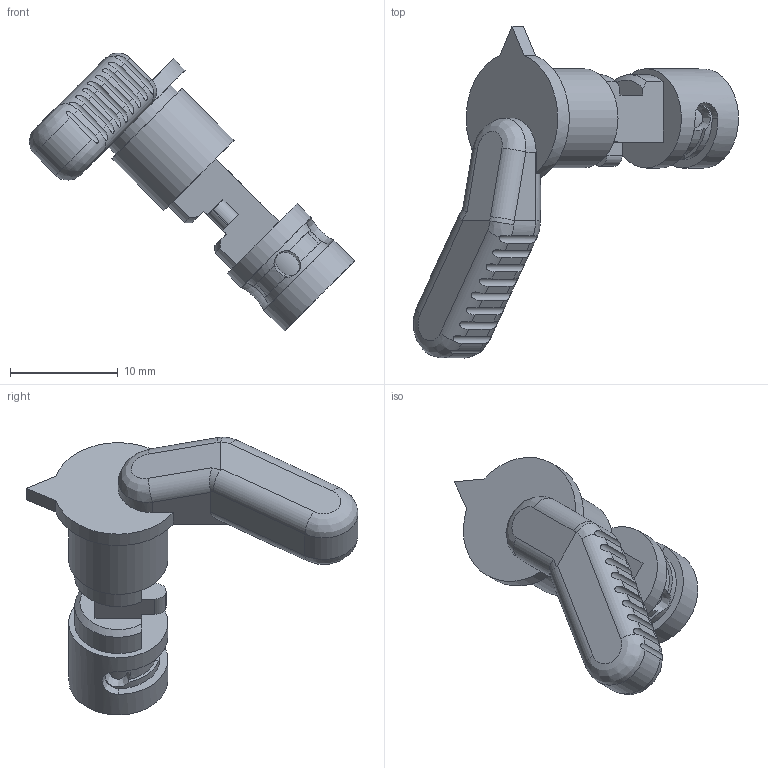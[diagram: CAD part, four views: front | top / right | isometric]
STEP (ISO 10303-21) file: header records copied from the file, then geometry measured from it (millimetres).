
FILE_DESCRIPTION(/* description */ (''),/* implementation_level */ '2;1');
FILE_NAME(/* name */ '',/* time_stamp */ '2021-12-08T23:04:14-05:00',/* author */ (''),/* organization */ (''),/* preprocessor_version */ 'ST-DEVELOPER v18.1',/* originating_system */ 'Autodesk Inventor 2022',/* authorisation */ '');
FILE_SCHEMA (('AUTOMOTIVE_DESIGN { 1 0 10303 214 3 1 1 }'));
Length unit declared in the file: inch
Products named in the file (1): ChoosyBoogleSelectorHK
Bounding box: 30.13 x 30.76 x 25.76 mm (x, y, z)
Volume: 2066.2 mm3; surface area: 1533 mm2
Topology: 1 solids, 1 shells, 92 faces, 247 edges, 162 vertices
Faces by surface type: plane 40, cylinder 38, bspline 11, cone 3
Full cylindrical faces by diameter (mm): 8.1 x1, 9.2 x2
Entity records: 3977 total; most frequent: CARTESIAN_POINT 1669, ORIENTED_EDGE 494, DIRECTION 436, EDGE_CURVE 247, VERTEX_POINT 162, AXIS2_PLACEMENT_3D 159, LINE 118, VECTOR 118
